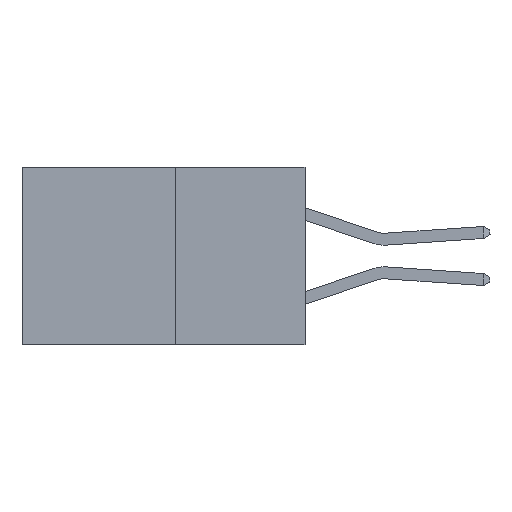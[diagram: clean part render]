
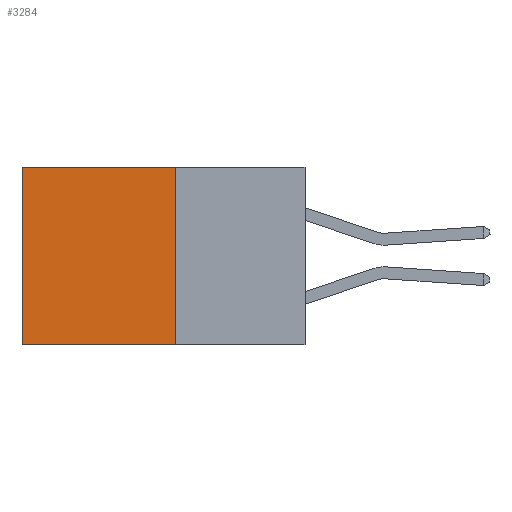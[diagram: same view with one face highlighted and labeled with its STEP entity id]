
A CAD part, left-side view. The second image highlights one B-rep face of the part: STEP entity #3284.
In plain terms, the highlighted planar face has unit normal (-1, 0, 0).
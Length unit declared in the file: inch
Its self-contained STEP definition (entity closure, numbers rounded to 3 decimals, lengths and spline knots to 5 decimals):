
#666 = LINE ( 'NONE', #2853, #4409 ) ;
#1766 = VERTEX_POINT ( 'NONE', #6449 ) ;
#1916 = CARTESIAN_POINT ( 'NONE',  ( 0.277, 0.59, -0.37 ) ) ;
#1926 = DIRECTION ( 'NONE',  ( 0., 1., 0. ) ) ;
#1980 = CARTESIAN_POINT ( 'NONE',  ( 0.277, 0.27, 0. ) ) ;
#2008 = EDGE_CURVE ( 'NONE', #1766, #3532, #7899, .T. ) ;
#2043 = VERTEX_POINT ( 'NONE', #5073 ) ;
#2424 = LINE ( 'NONE', #1980, #4181 ) ;
#2485 = VERTEX_POINT ( 'NONE', #3517 ) ;
#2495 = DIRECTION ( 'NONE',  ( 0., 0., -1. ) ) ;
#2654 = ORIENTED_EDGE ( 'NONE', *, *, #9287, .T. ) ;
#2700 = DIRECTION ( 'NONE',  ( 0., 0., -1. ) ) ;
#2853 = CARTESIAN_POINT ( 'NONE',  ( 0.277, 0.27, -0.37 ) ) ;
#3284 = ADVANCED_FACE ( 'NONE', ( #6640 ), #8486, .F. ) ;
#3310 = EDGE_CURVE ( 'NONE', #2043, #3532, #8315, .T. ) ;
#3311 = CARTESIAN_POINT ( 'NONE',  ( 0.277, 0.59, -0.37 ) ) ;
#3471 = EDGE_LOOP ( 'NONE', ( #9418, #3694, #4049, #2654 ) ) ;
#3517 = CARTESIAN_POINT ( 'NONE',  ( 0.277, 0.27, 0. ) ) ;
#3532 = VERTEX_POINT ( 'NONE', #1916 ) ;
#3648 = CARTESIAN_POINT ( 'NONE',  ( 0.277, 0.27, -0.37 ) ) ;
#3694 = ORIENTED_EDGE ( 'NONE', *, *, #2008, .F. ) ;
#3798 = DIRECTION ( 'NONE',  ( 0., 0., -1. ) ) ;
#3804 = DIRECTION ( 'NONE',  ( 1., 0., 0. ) ) ;
#4049 = ORIENTED_EDGE ( 'NONE', *, *, #9260, .F. ) ;
#4181 = VECTOR ( 'NONE', #1926, 39.37008 ) ;
#4409 = VECTOR ( 'NONE', #2495, 39.37008 ) ;
#5073 = CARTESIAN_POINT ( 'NONE',  ( 0.277, 0.59, 0. ) ) ;
#5513 = DIRECTION ( 'NONE',  ( 0., 1., 0. ) ) ;
#5966 = VECTOR ( 'NONE', #5513, 39.37008 ) ;
#6406 = VECTOR ( 'NONE', #2700, 39.37008 ) ;
#6449 = CARTESIAN_POINT ( 'NONE',  ( 0.277, 0.27, -0.37 ) ) ;
#6640 = FACE_OUTER_BOUND ( 'NONE', #3471, .T. ) ;
#7359 = AXIS2_PLACEMENT_3D ( 'NONE', #8111, #3804, #3798 ) ;
#7899 = LINE ( 'NONE', #3648, #5966 ) ;
#8111 = CARTESIAN_POINT ( 'NONE',  ( 0.277, 0.27, -0.37 ) ) ;
#8315 = LINE ( 'NONE', #3311, #6406 ) ;
#8486 = PLANE ( 'NONE',  #7359 ) ;
#9260 = EDGE_CURVE ( 'NONE', #2485, #1766, #666, .T. ) ;
#9287 = EDGE_CURVE ( 'NONE', #2485, #2043, #2424, .T. ) ;
#9418 = ORIENTED_EDGE ( 'NONE', *, *, #3310, .T. ) ;
